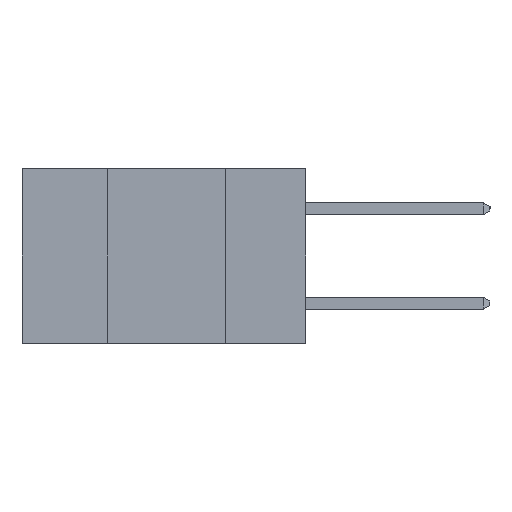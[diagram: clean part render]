
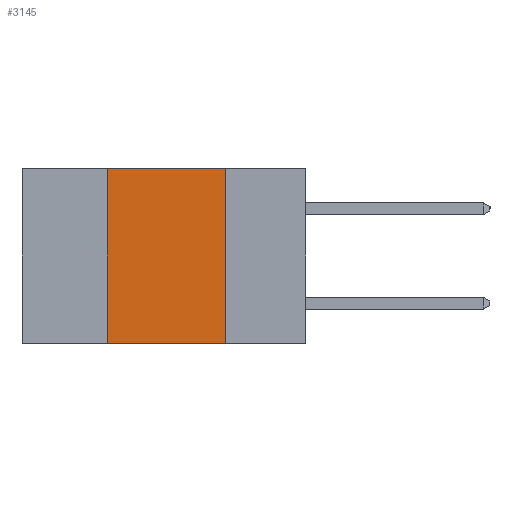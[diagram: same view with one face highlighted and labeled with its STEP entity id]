
A CAD part, left-side view. The second image highlights one B-rep face of the part: STEP entity #3145.
In plain terms, the highlighted planar face has unit normal (-1, 0, 0).
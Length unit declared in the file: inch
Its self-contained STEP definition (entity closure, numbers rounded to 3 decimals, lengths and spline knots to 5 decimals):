
#110 = CARTESIAN_POINT ( 'NONE',  ( 0., 0.42, -0.37 ) ) ;
#179 = CARTESIAN_POINT ( 'NONE',  ( 0., 0.17, -0.37 ) ) ;
#241 = EDGE_CURVE ( 'NONE', #5545, #1162, #7570, .T. ) ;
#317 = EDGE_CURVE ( 'NONE', #5545, #1423, #9083, .T. ) ;
#810 = DIRECTION ( 'NONE',  ( 0., -1., 0. ) ) ;
#906 = CARTESIAN_POINT ( 'NONE',  ( 0., 0.6, 0. ) ) ;
#946 = LINE ( 'NONE', #906, #7485 ) ;
#1162 = VERTEX_POINT ( 'NONE', #7723 ) ;
#1185 = CARTESIAN_POINT ( 'NONE',  ( 0., 0.6, 0. ) ) ;
#1191 = CARTESIAN_POINT ( 'NONE',  ( 0., 0.17, -0.37 ) ) ;
#1195 = EDGE_CURVE ( 'NONE', #1162, #3724, #946, .T. ) ;
#1423 = VERTEX_POINT ( 'NONE', #1191 ) ;
#2001 = DIRECTION ( 'NONE',  ( 0., 0., -1. ) ) ;
#2057 = CARTESIAN_POINT ( 'NONE',  ( 0., 0.42, -0.37 ) ) ;
#2238 = VECTOR ( 'NONE', #7659, 39.37008 ) ;
#2309 = DIRECTION ( 'NONE',  ( 0., 0., 1. ) ) ;
#2780 = VECTOR ( 'NONE', #5478, 39.37008 ) ;
#3145 = ADVANCED_FACE ( 'NONE', ( #5752 ), #8744, .F. ) ;
#3372 = ORIENTED_EDGE ( 'NONE', *, *, #3810, .F. ) ;
#3724 = VERTEX_POINT ( 'NONE', #4500 ) ;
#3810 = EDGE_CURVE ( 'NONE', #3724, #1423, #6882, .T. ) ;
#3971 = ORIENTED_EDGE ( 'NONE', *, *, #317, .T. ) ;
#4217 = DIRECTION ( 'NONE',  ( 1., 0., 0. ) ) ;
#4500 = CARTESIAN_POINT ( 'NONE',  ( 0., 0.17, 0. ) ) ;
#5478 = DIRECTION ( 'NONE',  ( 0., 0., -1. ) ) ;
#5545 = VERTEX_POINT ( 'NONE', #2057 ) ;
#5582 = VECTOR ( 'NONE', #2309, 39.37008 ) ;
#5752 = FACE_OUTER_BOUND ( 'NONE', #7891, .T. ) ;
#6882 = LINE ( 'NONE', #179, #2780 ) ;
#6886 = ORIENTED_EDGE ( 'NONE', *, *, #1195, .F. ) ;
#7485 = VECTOR ( 'NONE', #810, 39.37008 ) ;
#7570 = LINE ( 'NONE', #110, #5582 ) ;
#7659 = DIRECTION ( 'NONE',  ( 0., -1., 0. ) ) ;
#7723 = CARTESIAN_POINT ( 'NONE',  ( 0., 0.42, 0. ) ) ;
#7891 = EDGE_LOOP ( 'NONE', ( #3372, #6886, #8553, #3971 ) ) ;
#8553 = ORIENTED_EDGE ( 'NONE', *, *, #241, .F. ) ;
#8744 = PLANE ( 'NONE',  #9522 ) ;
#9083 = LINE ( 'NONE', #9176, #2238 ) ;
#9176 = CARTESIAN_POINT ( 'NONE',  ( 0., 0.6, -0.37 ) ) ;
#9522 = AXIS2_PLACEMENT_3D ( 'NONE', #1185, #4217, #2001 ) ;
